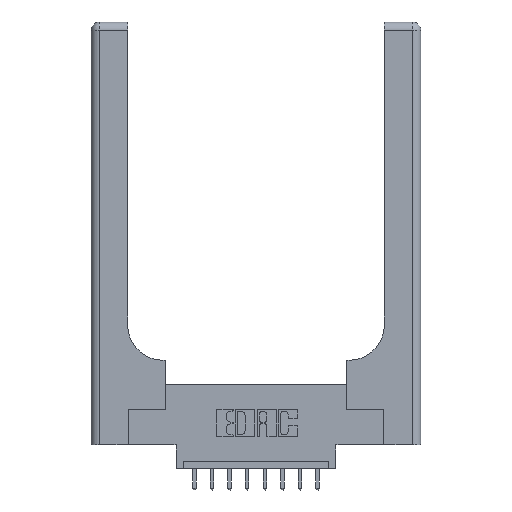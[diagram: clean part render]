
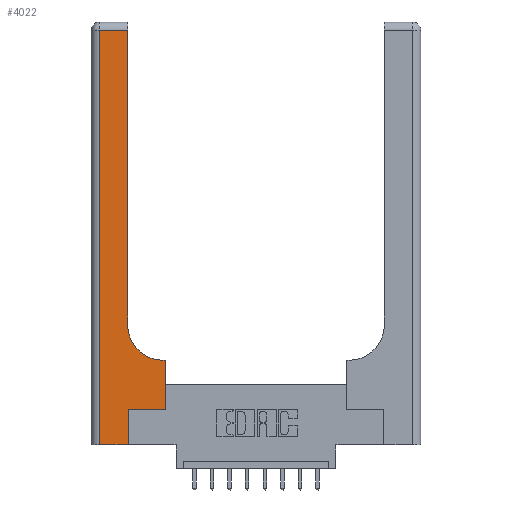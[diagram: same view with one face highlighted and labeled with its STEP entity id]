
A CAD part, top view. The second image highlights one B-rep face of the part: STEP entity #4022.
In plain terms, the highlighted planar face has unit normal (0, 0, 1).
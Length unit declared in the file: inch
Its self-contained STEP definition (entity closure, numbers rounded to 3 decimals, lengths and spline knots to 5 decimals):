
#187 = CARTESIAN_POINT ( 'NONE',  ( 0.26, 3., 0.37 ) ) ;
#362 = CARTESIAN_POINT ( 'NONE',  ( 0.528, 0.25, 0.37 ) ) ;
#643 = EDGE_CURVE ( 'NONE', #8855, #5234, #12738, .T. ) ;
#1138 = ORIENTED_EDGE ( 'NONE', *, *, #9909, .T. ) ;
#1354 = ORIENTED_EDGE ( 'NONE', *, *, #12641, .T. ) ;
#1570 = DIRECTION ( 'NONE',  ( 1., 0., 0. ) ) ;
#1579 = EDGE_CURVE ( 'NONE', #8825, #7245, #9637, .T. ) ;
#1966 = CIRCLE ( 'NONE', #5689, 0.25 ) ;
#2300 = CARTESIAN_POINT ( 'NONE',  ( 0.06, 2.94, 0.37 ) ) ;
#2670 = DIRECTION ( 'NONE',  ( 1., 0., 0. ) ) ;
#2851 = CARTESIAN_POINT ( 'NONE',  ( 0.528, 0.25, 0.37 ) ) ;
#3015 = DIRECTION ( 'NONE',  ( 0., -1., 0. ) ) ;
#3058 = VECTOR ( 'NONE', #1570, 39.37008 ) ;
#3225 = ORIENTED_EDGE ( 'NONE', *, *, #4626, .T. ) ;
#3315 = CARTESIAN_POINT ( 'NONE',  ( 0.06, 0., 0.37 ) ) ;
#3380 = DIRECTION ( 'NONE',  ( 0., 1., 0. ) ) ;
#3548 = DIRECTION ( 'NONE',  ( 1., 0., 0. ) ) ;
#3614 = VERTEX_POINT ( 'NONE', #13619 ) ;
#3786 = CARTESIAN_POINT ( 'NONE',  ( 0.51, 0.6, 0.37 ) ) ;
#3854 = DIRECTION ( 'NONE',  ( 0., 0., -1. ) ) ;
#3991 = VECTOR ( 'NONE', #4061, 39.37008 ) ;
#4022 = ADVANCED_FACE ( 'NONE', ( #6435 ), #5204, .F. ) ;
#4046 = EDGE_CURVE ( 'NONE', #13701, #5754, #11321, .T. ) ;
#4061 = DIRECTION ( 'NONE',  ( -1., 0., 0. ) ) ;
#4139 = VERTEX_POINT ( 'NONE', #6874 ) ;
#4163 = ORIENTED_EDGE ( 'NONE', *, *, #643, .T. ) ;
#4272 = ORIENTED_EDGE ( 'NONE', *, *, #9725, .T. ) ;
#4626 = EDGE_CURVE ( 'NONE', #5754, #3614, #7427, .T. ) ;
#4938 = LINE ( 'NONE', #9400, #6181 ) ;
#5108 = DIRECTION ( 'NONE',  ( 0., 1., 0. ) ) ;
#5204 = PLANE ( 'NONE',  #7843 ) ;
#5234 = VERTEX_POINT ( 'NONE', #3786 ) ;
#5253 = LINE ( 'NONE', #362, #8667 ) ;
#5359 = CARTESIAN_POINT ( 'NONE',  ( 0.06, 3., 0.37 ) ) ;
#5689 = AXIS2_PLACEMENT_3D ( 'NONE', #13263, #3854, #2670 ) ;
#5740 = CARTESIAN_POINT ( 'NONE',  ( 0.26, 0.6, 0.37 ) ) ;
#5754 = VERTEX_POINT ( 'NONE', #3315 ) ;
#6050 = CARTESIAN_POINT ( 'NONE',  ( 0., 0., 0.37 ) ) ;
#6181 = VECTOR ( 'NONE', #3548, 39.37008 ) ;
#6435 = FACE_OUTER_BOUND ( 'NONE', #6659, .T. ) ;
#6514 = CARTESIAN_POINT ( 'NONE',  ( 0., 3., 0.37 ) ) ;
#6659 = EDGE_LOOP ( 'NONE', ( #13376, #7453, #9114, #3225, #13873, #4272, #1354, #4163, #1138 ) ) ;
#6874 = CARTESIAN_POINT ( 'NONE',  ( 0.265, 0.25, 0.37 ) ) ;
#7082 = LINE ( 'NONE', #15203, #7242 ) ;
#7242 = VECTOR ( 'NONE', #3380, 39.37008 ) ;
#7245 = VERTEX_POINT ( 'NONE', #9798 ) ;
#7272 = VERTEX_POINT ( 'NONE', #2851 ) ;
#7427 = LINE ( 'NONE', #6050, #3058 ) ;
#7453 = ORIENTED_EDGE ( 'NONE', *, *, #11833, .T. ) ;
#7843 = AXIS2_PLACEMENT_3D ( 'NONE', #6514, #11179, #12259 ) ;
#8208 = VECTOR ( 'NONE', #9559, 39.37008 ) ;
#8667 = VECTOR ( 'NONE', #5108, 39.37008 ) ;
#8825 = VERTEX_POINT ( 'NONE', #12458 ) ;
#8855 = VERTEX_POINT ( 'NONE', #12607 ) ;
#9114 = ORIENTED_EDGE ( 'NONE', *, *, #4046, .T. ) ;
#9400 = CARTESIAN_POINT ( 'NONE',  ( 0.265, 0.25, 0.37 ) ) ;
#9559 = DIRECTION ( 'NONE',  ( 0., 1., 0. ) ) ;
#9637 = LINE ( 'NONE', #187, #8208 ) ;
#9725 = EDGE_CURVE ( 'NONE', #4139, #7272, #4938, .T. ) ;
#9798 = CARTESIAN_POINT ( 'NONE',  ( 0.26, 2.94, 0.37 ) ) ;
#9898 = LINE ( 'NONE', #12430, #3991 ) ;
#9909 = EDGE_CURVE ( 'NONE', #5234, #8825, #1966, .T. ) ;
#11179 = DIRECTION ( 'NONE',  ( 0., 0., -1. ) ) ;
#11321 = LINE ( 'NONE', #5359, #13744 ) ;
#11833 = EDGE_CURVE ( 'NONE', #7245, #13701, #9898, .T. ) ;
#12259 = DIRECTION ( 'NONE',  ( -1., 0., 0. ) ) ;
#12430 = CARTESIAN_POINT ( 'NONE',  ( 0., 2.94, 0.37 ) ) ;
#12458 = CARTESIAN_POINT ( 'NONE',  ( 0.26, 0.85, 0.37 ) ) ;
#12607 = CARTESIAN_POINT ( 'NONE',  ( 0.528, 0.6, 0.37 ) ) ;
#12641 = EDGE_CURVE ( 'NONE', #7272, #8855, #5253, .T. ) ;
#12738 = LINE ( 'NONE', #5740, #12858 ) ;
#12858 = VECTOR ( 'NONE', #15089, 39.37008 ) ;
#13263 = CARTESIAN_POINT ( 'NONE',  ( 0.51, 0.85, 0.37 ) ) ;
#13376 = ORIENTED_EDGE ( 'NONE', *, *, #1579, .T. ) ;
#13619 = CARTESIAN_POINT ( 'NONE',  ( 0.265, 0., 0.37 ) ) ;
#13701 = VERTEX_POINT ( 'NONE', #2300 ) ;
#13744 = VECTOR ( 'NONE', #3015, 39.37008 ) ;
#13873 = ORIENTED_EDGE ( 'NONE', *, *, #14893, .T. ) ;
#14893 = EDGE_CURVE ( 'NONE', #3614, #4139, #7082, .T. ) ;
#15089 = DIRECTION ( 'NONE',  ( -1., 0., 0. ) ) ;
#15203 = CARTESIAN_POINT ( 'NONE',  ( 0.265, 0., 0.37 ) ) ;
